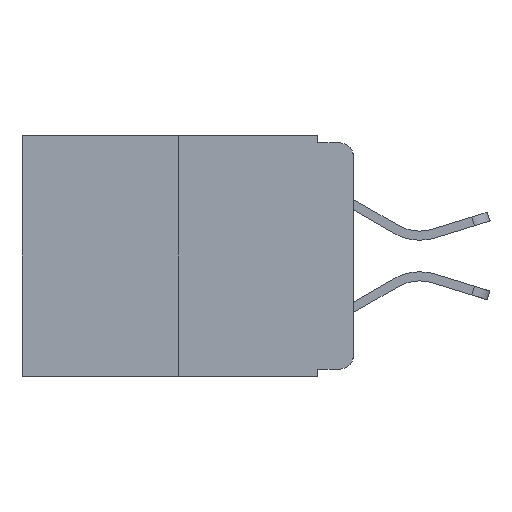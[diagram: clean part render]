
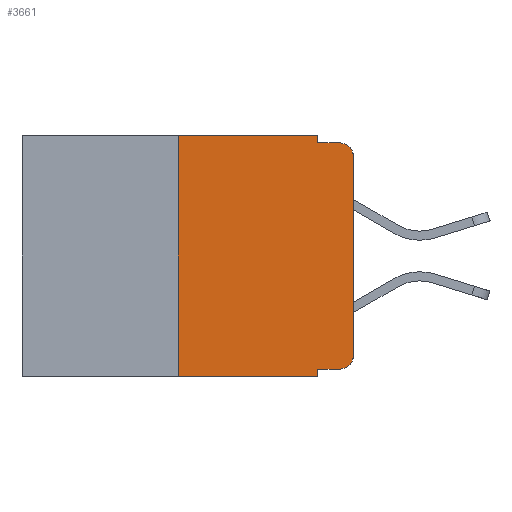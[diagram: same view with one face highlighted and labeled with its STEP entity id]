
A CAD part, left-side view. The second image highlights one B-rep face of the part: STEP entity #3661.
In plain terms, the highlighted planar face has unit normal (-1, 0, 0).
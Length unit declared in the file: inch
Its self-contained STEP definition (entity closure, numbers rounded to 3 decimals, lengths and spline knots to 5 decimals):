
#6 = LINE ( 'NONE', #9376, #2032 ) ;
#130 = VECTOR ( 'NONE', #3831, 39.37008 ) ;
#260 = VERTEX_POINT ( 'NONE', #9718 ) ;
#263 = ORIENTED_EDGE ( 'NONE', *, *, #4594, .T. ) ;
#392 = DIRECTION ( 'NONE',  ( 0., 0., -1. ) ) ;
#461 = EDGE_CURVE ( 'NONE', #2578, #260, #6, .T. ) ;
#468 = VECTOR ( 'NONE', #3885, 39.37008 ) ;
#562 = FACE_OUTER_BOUND ( 'NONE', #3029, .T. ) ;
#573 = CARTESIAN_POINT ( 'NONE',  ( 0., 0.051, -0.01 ) ) ;
#675 = CARTESIAN_POINT ( 'NONE',  ( 0., 0.473, 0. ) ) ;
#821 = EDGE_CURVE ( 'NONE', #8843, #7043, #4179, .T. ) ;
#936 = CARTESIAN_POINT ( 'NONE',  ( 0., 0., -0.03 ) ) ;
#981 = VERTEX_POINT ( 'NONE', #3655 ) ;
#1328 = VERTEX_POINT ( 'NONE', #2044 ) ;
#1393 = LINE ( 'NONE', #573, #468 ) ;
#1464 = DIRECTION ( 'NONE',  ( 0., 0., 1. ) ) ;
#1793 = AXIS2_PLACEMENT_3D ( 'NONE', #3148, #10457, #8903 ) ;
#1858 = LINE ( 'NONE', #7732, #9051 ) ;
#1901 = VERTEX_POINT ( 'NONE', #6179 ) ;
#1908 = ORIENTED_EDGE ( 'NONE', *, *, #5887, .F. ) ;
#1927 = EDGE_CURVE ( 'NONE', #2614, #2658, #5372, .T. ) ;
#1942 = ORIENTED_EDGE ( 'NONE', *, *, #2010, .F. ) ;
#2010 = EDGE_CURVE ( 'NONE', #981, #1901, #1393, .T. ) ;
#2032 = VECTOR ( 'NONE', #8361, 39.37008 ) ;
#2044 = CARTESIAN_POINT ( 'NONE',  ( 0., 0.25, 0. ) ) ;
#2170 = ORIENTED_EDGE ( 'NONE', *, *, #3830, .F. ) ;
#2265 = CARTESIAN_POINT ( 'NONE',  ( 0., 0.051, 0. ) ) ;
#2440 = CARTESIAN_POINT ( 'NONE',  ( 0., 0.051, 0. ) ) ;
#2578 = VERTEX_POINT ( 'NONE', #10645 ) ;
#2614 = VERTEX_POINT ( 'NONE', #9036 ) ;
#2658 = VERTEX_POINT ( 'NONE', #936 ) ;
#2954 = CARTESIAN_POINT ( 'NONE',  ( 0., 0., 0. ) ) ;
#2966 = VERTEX_POINT ( 'NONE', #2440 ) ;
#3029 = EDGE_LOOP ( 'NONE', ( #4335, #263, #1942, #8491, #2170, #1908, #5735, #7289, #8245, #9625 ) ) ;
#3063 = VECTOR ( 'NONE', #4007, 39.37008 ) ;
#3134 = LINE ( 'NONE', #2265, #3063 ) ;
#3148 = CARTESIAN_POINT ( 'NONE',  ( 0., 0.02, -0.03 ) ) ;
#3341 = AXIS2_PLACEMENT_3D ( 'NONE', #3873, #7157, #4509 ) ;
#3576 = AXIS2_PLACEMENT_3D ( 'NONE', #3777, #10334, #7390 ) ;
#3655 = CARTESIAN_POINT ( 'NONE',  ( 0., 0.051, -0.01 ) ) ;
#3661 = ADVANCED_FACE ( 'NONE', ( #562 ), #4612, .F. ) ;
#3777 = CARTESIAN_POINT ( 'NONE',  ( 0., 0.02, -0.313 ) ) ;
#3830 = EDGE_CURVE ( 'NONE', #1328, #2966, #4154, .T. ) ;
#3831 = DIRECTION ( 'NONE',  ( 0., 0., 1. ) ) ;
#3873 = CARTESIAN_POINT ( 'NONE',  ( 0., 0.473, 0. ) ) ;
#3885 = DIRECTION ( 'NONE',  ( 0., -1., 0. ) ) ;
#4007 = DIRECTION ( 'NONE',  ( 0., 0., -1. ) ) ;
#4154 = LINE ( 'NONE', #675, #10559 ) ;
#4179 = LINE ( 'NONE', #6524, #5095 ) ;
#4262 = CARTESIAN_POINT ( 'NONE',  ( 0., 0.25, -0.343 ) ) ;
#4272 = CIRCLE ( 'NONE', #3576, 0.02 ) ;
#4335 = ORIENTED_EDGE ( 'NONE', *, *, #1927, .T. ) ;
#4509 = DIRECTION ( 'NONE',  ( 0., 0., -1. ) ) ;
#4594 = EDGE_CURVE ( 'NONE', #2658, #1901, #10215, .T. ) ;
#4612 = PLANE ( 'NONE',  #3341 ) ;
#4762 = EDGE_CURVE ( 'NONE', #2966, #981, #1858, .T. ) ;
#4801 = CARTESIAN_POINT ( 'NONE',  ( 0., 0.25, 0. ) ) ;
#5095 = VECTOR ( 'NONE', #6629, 39.37008 ) ;
#5372 = LINE ( 'NONE', #2954, #130 ) ;
#5735 = ORIENTED_EDGE ( 'NONE', *, *, #821, .T. ) ;
#5887 = EDGE_CURVE ( 'NONE', #8843, #1328, #7182, .T. ) ;
#6179 = CARTESIAN_POINT ( 'NONE',  ( 0., 0.02, -0.01 ) ) ;
#6524 = CARTESIAN_POINT ( 'NONE',  ( 0., 0.473, -0.343 ) ) ;
#6629 = DIRECTION ( 'NONE',  ( 0., -1., 0. ) ) ;
#7043 = VERTEX_POINT ( 'NONE', #7186 ) ;
#7157 = DIRECTION ( 'NONE',  ( 1., 0., 0. ) ) ;
#7182 = LINE ( 'NONE', #4801, #9884 ) ;
#7186 = CARTESIAN_POINT ( 'NONE',  ( 0., 0.051, -0.343 ) ) ;
#7289 = ORIENTED_EDGE ( 'NONE', *, *, #7455, .F. ) ;
#7390 = DIRECTION ( 'NONE',  ( 0., 0., -1. ) ) ;
#7455 = EDGE_CURVE ( 'NONE', #2578, #7043, #3134, .T. ) ;
#7554 = EDGE_CURVE ( 'NONE', #260, #2614, #4272, .T. ) ;
#7732 = CARTESIAN_POINT ( 'NONE',  ( 0., 0.051, 0. ) ) ;
#8245 = ORIENTED_EDGE ( 'NONE', *, *, #461, .T. ) ;
#8361 = DIRECTION ( 'NONE',  ( 0., -1., 0. ) ) ;
#8491 = ORIENTED_EDGE ( 'NONE', *, *, #4762, .F. ) ;
#8843 = VERTEX_POINT ( 'NONE', #4262 ) ;
#8903 = DIRECTION ( 'NONE',  ( 0., 0., -1. ) ) ;
#9036 = CARTESIAN_POINT ( 'NONE',  ( 0., 0., -0.313 ) ) ;
#9051 = VECTOR ( 'NONE', #392, 39.37008 ) ;
#9376 = CARTESIAN_POINT ( 'NONE',  ( 0., 0.051, -0.333 ) ) ;
#9625 = ORIENTED_EDGE ( 'NONE', *, *, #7554, .T. ) ;
#9718 = CARTESIAN_POINT ( 'NONE',  ( 0., 0.02, -0.333 ) ) ;
#9884 = VECTOR ( 'NONE', #1464, 39.37008 ) ;
#10087 = DIRECTION ( 'NONE',  ( 0., -1., 0. ) ) ;
#10215 = CIRCLE ( 'NONE', #1793, 0.02 ) ;
#10334 = DIRECTION ( 'NONE',  ( -1., 0., 0. ) ) ;
#10457 = DIRECTION ( 'NONE',  ( -1., 0., 0. ) ) ;
#10559 = VECTOR ( 'NONE', #10087, 39.37008 ) ;
#10645 = CARTESIAN_POINT ( 'NONE',  ( 0., 0.051, -0.333 ) ) ;
